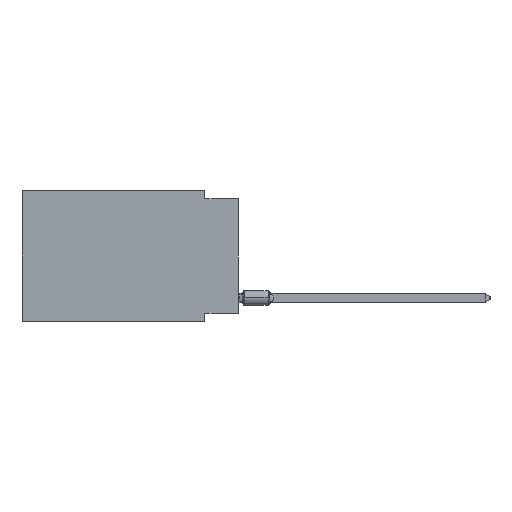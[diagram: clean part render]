
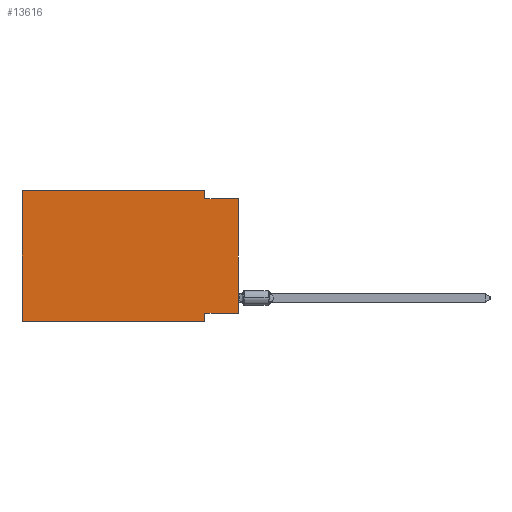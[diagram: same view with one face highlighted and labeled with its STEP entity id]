
A CAD part, left-side view. The second image highlights one B-rep face of the part: STEP entity #13616.
In plain terms, the highlighted planar face has unit normal (-1, 0, 0).
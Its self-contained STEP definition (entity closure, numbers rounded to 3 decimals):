
#531 = VECTOR ( 'NONE', #28759, 1000. ) ;
#1060 = EDGE_CURVE ( 'NONE', #5065, #8387, #12750, .T. ) ;
#1667 = EDGE_CURVE ( 'NONE', #14436, #28750, #33798, .T. ) ;
#1711 = CARTESIAN_POINT ( 'NONE',  ( 0., 16.383, 0. ) ) ;
#3577 = ORIENTED_EDGE ( 'NONE', *, *, #5860, .F. ) ;
#4474 = VERTEX_POINT ( 'NONE', #1711 ) ;
#5065 = VERTEX_POINT ( 'NONE', #6404 ) ;
#5127 = LINE ( 'NONE', #27570, #30544 ) ;
#5179 = ORIENTED_EDGE ( 'NONE', *, *, #23964, .F. ) ;
#5860 = EDGE_CURVE ( 'NONE', #32514, #4474, #29059, .T. ) ;
#6404 = CARTESIAN_POINT ( 'NONE',  ( 0., 2.54, 0. ) ) ;
#6437 = VECTOR ( 'NONE', #26776, 1000. ) ;
#7015 = CARTESIAN_POINT ( 'NONE',  ( 0., 0., -9.271 ) ) ;
#7546 = PLANE ( 'NONE',  #26136 ) ;
#8387 = VERTEX_POINT ( 'NONE', #33837 ) ;
#8757 = EDGE_LOOP ( 'NONE', ( #10950, #5179, #11940, #23681, #3577, #11687, #34632, #18693 ) ) ;
#8959 = CARTESIAN_POINT ( 'NONE',  ( 0., 16.383, -9.906 ) ) ;
#9759 = LINE ( 'NONE', #7015, #20486 ) ;
#10387 = LINE ( 'NONE', #21496, #31294 ) ;
#10631 = FACE_OUTER_BOUND ( 'NONE', #8757, .T. ) ;
#10950 = ORIENTED_EDGE ( 'NONE', *, *, #1667, .T. ) ;
#11687 = ORIENTED_EDGE ( 'NONE', *, *, #17876, .T. ) ;
#11910 = VECTOR ( 'NONE', #23242, 1000. ) ;
#11940 = ORIENTED_EDGE ( 'NONE', *, *, #1060, .F. ) ;
#12750 = LINE ( 'NONE', #15665, #6437 ) ;
#13562 = CARTESIAN_POINT ( 'NONE',  ( 0., 16.383, 0. ) ) ;
#13616 = ADVANCED_FACE ( 'NONE', ( #10631 ), #7546, .F. ) ;
#14436 = VERTEX_POINT ( 'NONE', #31762 ) ;
#14737 = LINE ( 'NONE', #15094, #531 ) ;
#15094 = CARTESIAN_POINT ( 'NONE',  ( 0., 16.383, -9.906 ) ) ;
#15665 = CARTESIAN_POINT ( 'NONE',  ( 0., 2.54, 0. ) ) ;
#17876 = EDGE_CURVE ( 'NONE', #32514, #19865, #14737, .T. ) ;
#18667 = DIRECTION ( 'NONE',  ( 0., 0., -1. ) ) ;
#18693 = ORIENTED_EDGE ( 'NONE', *, *, #31891, .F. ) ;
#18961 = CARTESIAN_POINT ( 'NONE',  ( 0., 2.54, -9.906 ) ) ;
#19777 = DIRECTION ( 'NONE',  ( 0., 0., 1. ) ) ;
#19865 = VERTEX_POINT ( 'NONE', #18961 ) ;
#20486 = VECTOR ( 'NONE', #24154, 1000. ) ;
#20686 = CARTESIAN_POINT ( 'NONE',  ( 0., 16.383, 0. ) ) ;
#21496 = CARTESIAN_POINT ( 'NONE',  ( 0., 2.54, -9.906 ) ) ;
#22279 = CARTESIAN_POINT ( 'NONE',  ( 0., 0., -0.635 ) ) ;
#23242 = DIRECTION ( 'NONE',  ( 0., 0., 1. ) ) ;
#23681 = ORIENTED_EDGE ( 'NONE', *, *, #31795, .F. ) ;
#23964 = EDGE_CURVE ( 'NONE', #8387, #28750, #5127, .T. ) ;
#24154 = DIRECTION ( 'NONE',  ( 0., 1., 0. ) ) ;
#25269 = DIRECTION ( 'NONE',  ( 0., -1., 0. ) ) ;
#25457 = LINE ( 'NONE', #31283, #28057 ) ;
#26136 = AXIS2_PLACEMENT_3D ( 'NONE', #13562, #27586, #18667 ) ;
#26776 = DIRECTION ( 'NONE',  ( 0., 0., -1. ) ) ;
#27570 = CARTESIAN_POINT ( 'NONE',  ( 0., 0., -0.635 ) ) ;
#27586 = DIRECTION ( 'NONE',  ( 1., 0., 0. ) ) ;
#27973 = CARTESIAN_POINT ( 'NONE',  ( 0., 0., 0. ) ) ;
#28057 = VECTOR ( 'NONE', #25269, 1000. ) ;
#28750 = VERTEX_POINT ( 'NONE', #22279 ) ;
#28759 = DIRECTION ( 'NONE',  ( 0., -1., 0. ) ) ;
#29059 = LINE ( 'NONE', #20686, #11910 ) ;
#29140 = VECTOR ( 'NONE', #19777, 1000. ) ;
#29564 = EDGE_CURVE ( 'NONE', #30236, #19865, #10387, .T. ) ;
#30236 = VERTEX_POINT ( 'NONE', #34507 ) ;
#30544 = VECTOR ( 'NONE', #35399, 1000. ) ;
#31283 = CARTESIAN_POINT ( 'NONE',  ( 0., 16.383, 0. ) ) ;
#31294 = VECTOR ( 'NONE', #32618, 1000. ) ;
#31762 = CARTESIAN_POINT ( 'NONE',  ( 0., 0., -9.271 ) ) ;
#31795 = EDGE_CURVE ( 'NONE', #4474, #5065, #25457, .T. ) ;
#31891 = EDGE_CURVE ( 'NONE', #14436, #30236, #9759, .T. ) ;
#32514 = VERTEX_POINT ( 'NONE', #8959 ) ;
#32618 = DIRECTION ( 'NONE',  ( 0., 0., -1. ) ) ;
#33798 = LINE ( 'NONE', #27973, #29140 ) ;
#33837 = CARTESIAN_POINT ( 'NONE',  ( 0., 2.54, -0.635 ) ) ;
#34507 = CARTESIAN_POINT ( 'NONE',  ( 0., 2.54, -9.271 ) ) ;
#34632 = ORIENTED_EDGE ( 'NONE', *, *, #29564, .F. ) ;
#35399 = DIRECTION ( 'NONE',  ( 0., -1., 0. ) ) ;
